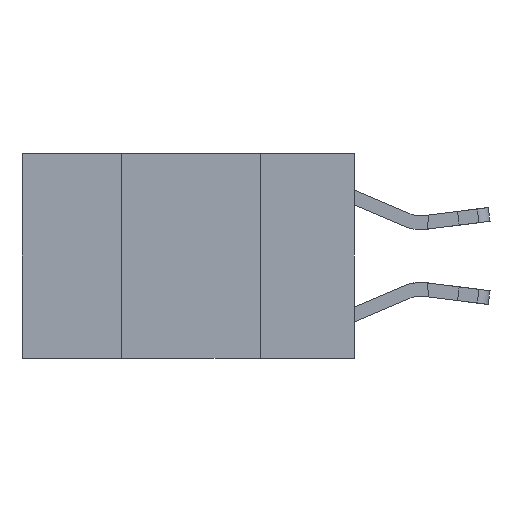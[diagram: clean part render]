
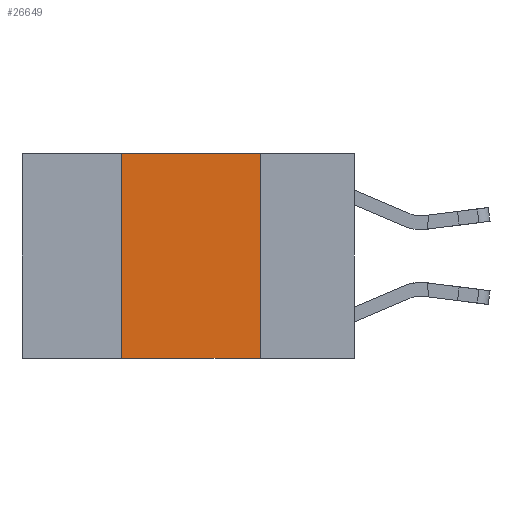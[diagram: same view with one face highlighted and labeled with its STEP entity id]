
A CAD part, left-side view. The second image highlights one B-rep face of the part: STEP entity #26649.
In plain terms, the highlighted planar face has unit normal (-1, 0, 0).
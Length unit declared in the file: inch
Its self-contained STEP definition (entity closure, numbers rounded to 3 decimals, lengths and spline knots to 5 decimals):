
#684 = EDGE_CURVE ( 'NONE', #6388, #21338, #25535, .T. ) ;
#685 = PLANE ( 'NONE',  #7150 ) ;
#768 = LINE ( 'NONE', #5439, #16265 ) ;
#4704 = DIRECTION ( 'NONE',  ( 0., -1., 0. ) ) ;
#5439 = CARTESIAN_POINT ( 'NONE',  ( 0., 0.42, 0. ) ) ;
#6388 = VERTEX_POINT ( 'NONE', #8605 ) ;
#6430 = VECTOR ( 'NONE', #14244, 39.37008 ) ;
#6736 = CARTESIAN_POINT ( 'NONE',  ( 0., 0.17, 0. ) ) ;
#7150 = AXIS2_PLACEMENT_3D ( 'NONE', #10019, #18792, #14239 ) ;
#7192 = CARTESIAN_POINT ( 'NONE',  ( 0., 0.17, -0.37 ) ) ;
#8605 = CARTESIAN_POINT ( 'NONE',  ( 0., 0.42, 0. ) ) ;
#9239 = CARTESIAN_POINT ( 'NONE',  ( 0., 0.17, 0. ) ) ;
#10019 = CARTESIAN_POINT ( 'NONE',  ( 0., 0.6, 0. ) ) ;
#10258 = DIRECTION ( 'NONE',  ( 0., 0., 1. ) ) ;
#12201 = FACE_OUTER_BOUND ( 'NONE', #26231, .T. ) ;
#13557 = EDGE_CURVE ( 'NONE', #17670, #6388, #768, .T. ) ;
#14239 = DIRECTION ( 'NONE',  ( 0., 0., -1. ) ) ;
#14244 = DIRECTION ( 'NONE',  ( 0., -1., 0. ) ) ;
#15374 = LINE ( 'NONE', #20442, #23248 ) ;
#15953 = DIRECTION ( 'NONE',  ( 0., 0., -1. ) ) ;
#16265 = VECTOR ( 'NONE', #10258, 39.37008 ) ;
#16462 = VERTEX_POINT ( 'NONE', #7192 ) ;
#16841 = EDGE_CURVE ( 'NONE', #17670, #16462, #15374, .T. ) ;
#17670 = VERTEX_POINT ( 'NONE', #26143 ) ;
#18496 = CARTESIAN_POINT ( 'NONE',  ( 0., 0.6, 0. ) ) ;
#18792 = DIRECTION ( 'NONE',  ( 1., 0., 0. ) ) ;
#19214 = VECTOR ( 'NONE', #15953, 39.37008 ) ;
#20442 = CARTESIAN_POINT ( 'NONE',  ( 0., 0.6, -0.37 ) ) ;
#21338 = VERTEX_POINT ( 'NONE', #6736 ) ;
#21412 = ORIENTED_EDGE ( 'NONE', *, *, #23862, .F. ) ;
#21416 = ORIENTED_EDGE ( 'NONE', *, *, #16841, .T. ) ;
#22700 = LINE ( 'NONE', #9239, #19214 ) ;
#23248 = VECTOR ( 'NONE', #4704, 39.37008 ) ;
#23257 = ORIENTED_EDGE ( 'NONE', *, *, #13557, .F. ) ;
#23862 = EDGE_CURVE ( 'NONE', #21338, #16462, #22700, .T. ) ;
#23954 = ORIENTED_EDGE ( 'NONE', *, *, #684, .F. ) ;
#25535 = LINE ( 'NONE', #18496, #6430 ) ;
#26143 = CARTESIAN_POINT ( 'NONE',  ( 0., 0.42, -0.37 ) ) ;
#26231 = EDGE_LOOP ( 'NONE', ( #21412, #23954, #23257, #21416 ) ) ;
#26649 = ADVANCED_FACE ( 'NONE', ( #12201 ), #685, .F. ) ;
